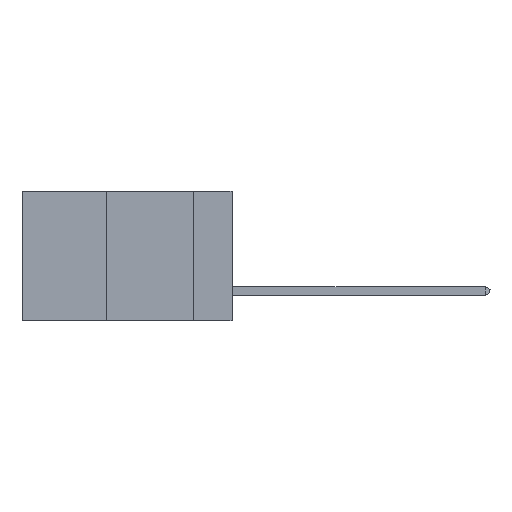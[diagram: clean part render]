
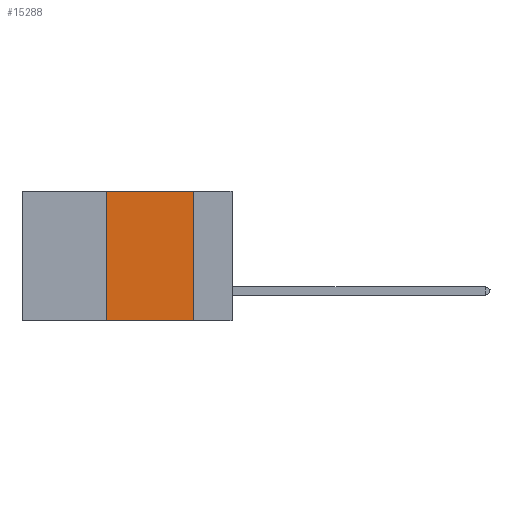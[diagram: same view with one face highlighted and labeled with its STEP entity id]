
A CAD part, left-side view. The second image highlights one B-rep face of the part: STEP entity #15288.
In plain terms, the highlighted planar face has unit normal (-1, 0, 0).
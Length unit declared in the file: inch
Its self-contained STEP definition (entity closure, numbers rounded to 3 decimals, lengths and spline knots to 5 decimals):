
#132 = VECTOR ( 'NONE', #13323, 39.37008 ) ;
#602 = VECTOR ( 'NONE', #13747, 39.37008 ) ;
#1163 = VECTOR ( 'NONE', #4175, 39.37008 ) ;
#1564 = AXIS2_PLACEMENT_3D ( 'NONE', #24234, #9371, #16800 ) ;
#2126 = LINE ( 'NONE', #18666, #602 ) ;
#2255 = EDGE_LOOP ( 'NONE', ( #2367, #22867, #19255, #25641 ) ) ;
#2307 = EDGE_CURVE ( 'NONE', #28159, #10156, #8931, .T. ) ;
#2367 = ORIENTED_EDGE ( 'NONE', *, *, #2307, .F. ) ;
#3568 = CARTESIAN_POINT ( 'NONE',  ( 0., 0.11, -0.37 ) ) ;
#4175 = DIRECTION ( 'NONE',  ( 0., 0., -1. ) ) ;
#6893 = PLANE ( 'NONE',  #1564 ) ;
#7140 = VERTEX_POINT ( 'NONE', #17872 ) ;
#7732 = LINE ( 'NONE', #10842, #17849 ) ;
#8885 = CARTESIAN_POINT ( 'NONE',  ( 0., 0.36, 0. ) ) ;
#8931 = LINE ( 'NONE', #24019, #1163 ) ;
#9371 = DIRECTION ( 'NONE',  ( 1., 0., 0. ) ) ;
#10156 = VERTEX_POINT ( 'NONE', #3568 ) ;
#10802 = EDGE_CURVE ( 'NONE', #21926, #28159, #7732, .T. ) ;
#10842 = CARTESIAN_POINT ( 'NONE',  ( 0., 0.6, 0. ) ) ;
#12031 = FACE_OUTER_BOUND ( 'NONE', #2255, .T. ) ;
#13323 = DIRECTION ( 'NONE',  ( 0., -1., 0. ) ) ;
#13747 = DIRECTION ( 'NONE',  ( 0., 0., 1. ) ) ;
#14935 = CARTESIAN_POINT ( 'NONE',  ( 0., 0.11, 0. ) ) ;
#15288 = ADVANCED_FACE ( 'NONE', ( #12031 ), #6893, .F. ) ;
#16800 = DIRECTION ( 'NONE',  ( 0., 0., -1. ) ) ;
#17849 = VECTOR ( 'NONE', #30516, 39.37008 ) ;
#17872 = CARTESIAN_POINT ( 'NONE',  ( 0., 0.36, -0.37 ) ) ;
#18666 = CARTESIAN_POINT ( 'NONE',  ( 0., 0.36, 0. ) ) ;
#19255 = ORIENTED_EDGE ( 'NONE', *, *, #28497, .F. ) ;
#21926 = VERTEX_POINT ( 'NONE', #8885 ) ;
#22867 = ORIENTED_EDGE ( 'NONE', *, *, #10802, .F. ) ;
#22992 = CARTESIAN_POINT ( 'NONE',  ( 0., 0.6, -0.37 ) ) ;
#24019 = CARTESIAN_POINT ( 'NONE',  ( 0., 0.11, 0. ) ) ;
#24171 = LINE ( 'NONE', #22992, #132 ) ;
#24234 = CARTESIAN_POINT ( 'NONE',  ( 0., 0.6, 0. ) ) ;
#25641 = ORIENTED_EDGE ( 'NONE', *, *, #30193, .T. ) ;
#28159 = VERTEX_POINT ( 'NONE', #14935 ) ;
#28497 = EDGE_CURVE ( 'NONE', #7140, #21926, #2126, .T. ) ;
#30193 = EDGE_CURVE ( 'NONE', #7140, #10156, #24171, .T. ) ;
#30516 = DIRECTION ( 'NONE',  ( 0., -1., 0. ) ) ;
